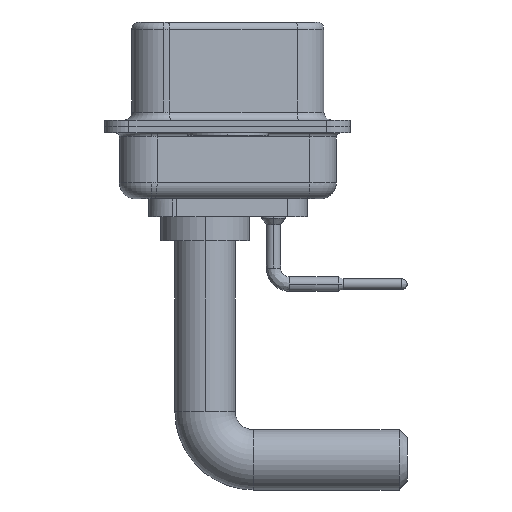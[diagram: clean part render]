
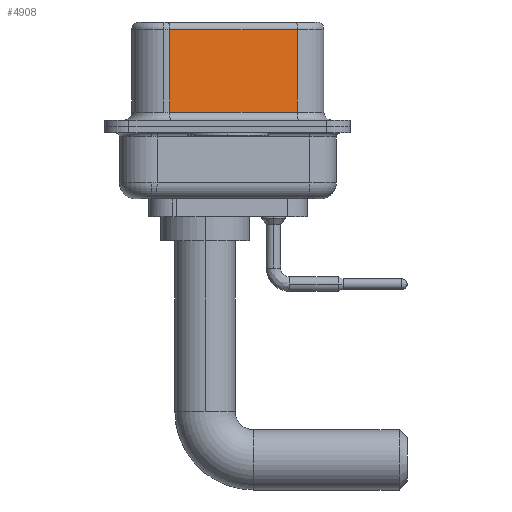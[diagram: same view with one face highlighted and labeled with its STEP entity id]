
A CAD part, left-side view. The second image highlights one B-rep face of the part: STEP entity #4908.
In plain terms, the highlighted planar face has unit normal (-0.985, -0.174, 0).
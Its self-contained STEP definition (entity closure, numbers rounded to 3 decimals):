
#233 = CARTESIAN_POINT ( 'NONE',  ( 3.73, 3.628, 0.9 ) ) ;
#565 = ORIENTED_EDGE ( 'NONE', *, *, #15388, .T. ) ;
#669 = CARTESIAN_POINT ( 'NONE',  ( 5.132, -4.322, 6.02 ) ) ;
#888 = LINE ( 'NONE', #669, #21978 ) ;
#1439 = FACE_OUTER_BOUND ( 'NONE', #20020, .T. ) ;
#2089 = ORIENTED_EDGE ( 'NONE', *, *, #11480, .T. ) ;
#2194 = VECTOR ( 'NONE', #20155, 1000. ) ;
#3519 = EDGE_CURVE ( 'NONE', #17328, #13349, #8950, .T. ) ;
#3831 = LINE ( 'NONE', #21035, #21824 ) ;
#4908 = ADVANCED_FACE ( 'NONE', ( #1439 ), #11729, .F. ) ;
#5736 = ORIENTED_EDGE ( 'NONE', *, *, #3519, .F. ) ;
#6353 = ORIENTED_EDGE ( 'NONE', *, *, #21684, .T. ) ;
#6686 = DIRECTION ( 'NONE',  ( -0.174, 0.985, 0. ) ) ;
#6794 = DIRECTION ( 'NONE',  ( 0.985, 0.174, 0. ) ) ;
#8950 = LINE ( 'NONE', #12213, #13352 ) ;
#9713 = VERTEX_POINT ( 'NONE', #15225 ) ;
#10199 = VERTEX_POINT ( 'NONE', #233 ) ;
#11480 = EDGE_CURVE ( 'NONE', #9713, #10199, #15229, .T. ) ;
#11729 = PLANE ( 'NONE',  #18419 ) ;
#12213 = CARTESIAN_POINT ( 'NONE',  ( 5.132, -4.322, 6.52 ) ) ;
#12972 = DIRECTION ( 'NONE',  ( 0.174, -0.985, 0. ) ) ;
#13348 = CARTESIAN_POINT ( 'NONE',  ( 3.73, 3.628, 6.52 ) ) ;
#13349 = VERTEX_POINT ( 'NONE', #14230 ) ;
#13352 = VECTOR ( 'NONE', #15867, 1000. ) ;
#13603 = CARTESIAN_POINT ( 'NONE',  ( 5.132, -4.322, 6.52 ) ) ;
#13682 = CARTESIAN_POINT ( 'NONE',  ( 5.132, -4.322, 6.02 ) ) ;
#14230 = CARTESIAN_POINT ( 'NONE',  ( 5.132, -4.322, 0.9 ) ) ;
#15225 = CARTESIAN_POINT ( 'NONE',  ( 3.73, 3.628, 6.02 ) ) ;
#15229 = LINE ( 'NONE', #13348, #2194 ) ;
#15388 = EDGE_CURVE ( 'NONE', #17328, #9713, #888, .T. ) ;
#15867 = DIRECTION ( 'NONE',  ( 0., 0., -1. ) ) ;
#17328 = VERTEX_POINT ( 'NONE', #13682 ) ;
#18419 = AXIS2_PLACEMENT_3D ( 'NONE', #13603, #6794, #6686 ) ;
#20020 = EDGE_LOOP ( 'NONE', ( #5736, #565, #2089, #6353 ) ) ;
#20155 = DIRECTION ( 'NONE',  ( 0., 0., -1. ) ) ;
#21035 = CARTESIAN_POINT ( 'NONE',  ( 5.132, -4.322, 0.9 ) ) ;
#21106 = DIRECTION ( 'NONE',  ( -0.174, 0.985, 0. ) ) ;
#21684 = EDGE_CURVE ( 'NONE', #10199, #13349, #3831, .T. ) ;
#21824 = VECTOR ( 'NONE', #12972, 1000. ) ;
#21978 = VECTOR ( 'NONE', #21106, 1000. ) ;
